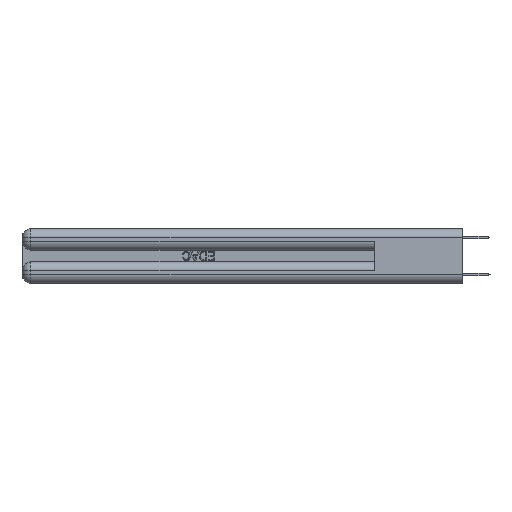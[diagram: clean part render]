
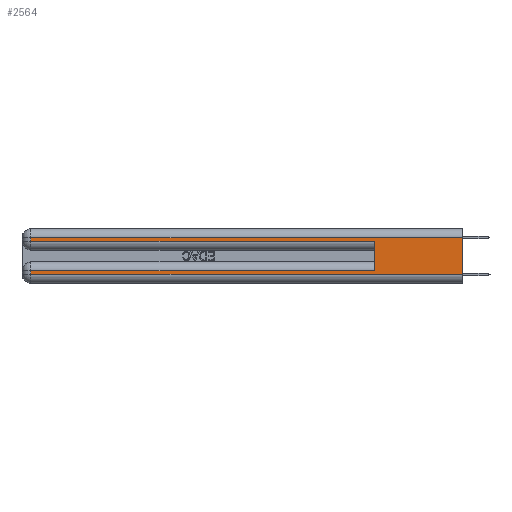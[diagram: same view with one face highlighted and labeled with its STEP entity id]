
A CAD part, left-side view. The second image highlights one B-rep face of the part: STEP entity #2564.
In plain terms, the highlighted planar face has unit normal (-1, 0, 0).
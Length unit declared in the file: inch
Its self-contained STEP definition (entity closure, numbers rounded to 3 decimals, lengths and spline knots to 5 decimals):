
#158 = EDGE_CURVE ( 'NONE', #3832, #15266, #17527, .T. ) ;
#1482 = VECTOR ( 'NONE', #22630, 39.37008 ) ;
#1990 = ORIENTED_EDGE ( 'NONE', *, *, #26379, .T. ) ;
#2042 = EDGE_CURVE ( 'NONE', #13567, #22661, #29156, .T. ) ;
#2335 = VECTOR ( 'NONE', #18645, 39.37008 ) ;
#2564 = ADVANCED_FACE ( 'NONE', ( #10258 ), #25598, .F. ) ;
#3832 = VERTEX_POINT ( 'NONE', #18506 ) ;
#4275 = CARTESIAN_POINT ( 'NONE',  ( 0., 2.94, 0.37 ) ) ;
#4915 = CARTESIAN_POINT ( 'NONE',  ( 0., 2.94, 0.285 ) ) ;
#5183 = DIRECTION ( 'NONE',  ( 0., -1., 0. ) ) ;
#6101 = VECTOR ( 'NONE', #5183, 39.37008 ) ;
#7601 = DIRECTION ( 'NONE',  ( 0., -1., 0. ) ) ;
#7924 = CARTESIAN_POINT ( 'NONE',  ( 0., 0., 0.06 ) ) ;
#8417 = DIRECTION ( 'NONE',  ( 0., 0., -1. ) ) ;
#8921 = ORIENTED_EDGE ( 'NONE', *, *, #158, .T. ) ;
#9600 = LINE ( 'NONE', #7924, #32822 ) ;
#9813 = VECTOR ( 'NONE', #26592, 39.37008 ) ;
#9955 = ORIENTED_EDGE ( 'NONE', *, *, #25597, .T. ) ;
#10258 = FACE_OUTER_BOUND ( 'NONE', #27561, .T. ) ;
#10584 = DIRECTION ( 'NONE',  ( 1., 0., 0. ) ) ;
#12056 = VECTOR ( 'NONE', #8417, 39.37008 ) ;
#12097 = CARTESIAN_POINT ( 'NONE',  ( 0., 0.6, 0.145 ) ) ;
#13051 = CARTESIAN_POINT ( 'NONE',  ( 0., 0., 0.285 ) ) ;
#13112 = AXIS2_PLACEMENT_3D ( 'NONE', #15020, #10584, #21118 ) ;
#13567 = VERTEX_POINT ( 'NONE', #25727 ) ;
#13587 = CARTESIAN_POINT ( 'NONE',  ( 0., 0., 0.06 ) ) ;
#14212 = ORIENTED_EDGE ( 'NONE', *, *, #2042, .T. ) ;
#15020 = CARTESIAN_POINT ( 'NONE',  ( 0., 0., 0.37 ) ) ;
#15266 = VERTEX_POINT ( 'NONE', #22102 ) ;
#15532 = DIRECTION ( 'NONE',  ( 0., 0., -1. ) ) ;
#15832 = LINE ( 'NONE', #16043, #2335 ) ;
#16043 = CARTESIAN_POINT ( 'NONE',  ( 0., 0., 0.31 ) ) ;
#16575 = VECTOR ( 'NONE', #28345, 39.37008 ) ;
#16823 = CARTESIAN_POINT ( 'NONE',  ( 0., 0., 0.31 ) ) ;
#17145 = VECTOR ( 'NONE', #15532, 39.37008 ) ;
#17527 = LINE ( 'NONE', #18475, #9813 ) ;
#18475 = CARTESIAN_POINT ( 'NONE',  ( 0., 0., 0.085 ) ) ;
#18506 = CARTESIAN_POINT ( 'NONE',  ( 0., 0.6, 0.085 ) ) ;
#18645 = DIRECTION ( 'NONE',  ( 0., 1., 0. ) ) ;
#19673 = CARTESIAN_POINT ( 'NONE',  ( 0., 2.94, 0.06 ) ) ;
#21118 = DIRECTION ( 'NONE',  ( 0., 0., -1. ) ) ;
#21160 = ORIENTED_EDGE ( 'NONE', *, *, #32319, .T. ) ;
#21704 = ORIENTED_EDGE ( 'NONE', *, *, #30904, .F. ) ;
#22102 = CARTESIAN_POINT ( 'NONE',  ( 0., 2.94, 0.085 ) ) ;
#22630 = DIRECTION ( 'NONE',  ( 0., 0., 1. ) ) ;
#22661 = VERTEX_POINT ( 'NONE', #4915 ) ;
#23438 = ORIENTED_EDGE ( 'NONE', *, *, #29400, .F. ) ;
#23822 = EDGE_CURVE ( 'NONE', #22661, #31273, #30614, .T. ) ;
#24074 = LINE ( 'NONE', #28565, #17145 ) ;
#25446 = VERTEX_POINT ( 'NONE', #19673 ) ;
#25534 = LINE ( 'NONE', #28579, #16575 ) ;
#25597 = EDGE_CURVE ( 'NONE', #27294, #13567, #15832, .T. ) ;
#25598 = PLANE ( 'NONE',  #13112 ) ;
#25727 = CARTESIAN_POINT ( 'NONE',  ( 0., 2.94, 0.31 ) ) ;
#26263 = CARTESIAN_POINT ( 'NONE',  ( 0., 0.6, 0.285 ) ) ;
#26379 = EDGE_CURVE ( 'NONE', #15266, #25446, #25534, .T. ) ;
#26592 = DIRECTION ( 'NONE',  ( 0., 1., 0. ) ) ;
#27294 = VERTEX_POINT ( 'NONE', #16823 ) ;
#27561 = EDGE_LOOP ( 'NONE', ( #23438, #9955, #14212, #30786, #21704, #8921, #1990, #21160 ) ) ;
#27651 = LINE ( 'NONE', #12097, #1482 ) ;
#28345 = DIRECTION ( 'NONE',  ( 0., 0., -1. ) ) ;
#28565 = CARTESIAN_POINT ( 'NONE',  ( 0., 0., 0.37 ) ) ;
#28579 = CARTESIAN_POINT ( 'NONE',  ( 0., 2.94, 0.37 ) ) ;
#29156 = LINE ( 'NONE', #4275, #12056 ) ;
#29400 = EDGE_CURVE ( 'NONE', #27294, #32423, #24074, .T. ) ;
#30614 = LINE ( 'NONE', #13051, #6101 ) ;
#30786 = ORIENTED_EDGE ( 'NONE', *, *, #23822, .T. ) ;
#30904 = EDGE_CURVE ( 'NONE', #3832, #31273, #27651, .T. ) ;
#31273 = VERTEX_POINT ( 'NONE', #26263 ) ;
#32319 = EDGE_CURVE ( 'NONE', #25446, #32423, #9600, .T. ) ;
#32423 = VERTEX_POINT ( 'NONE', #13587 ) ;
#32822 = VECTOR ( 'NONE', #7601, 39.37008 ) ;
